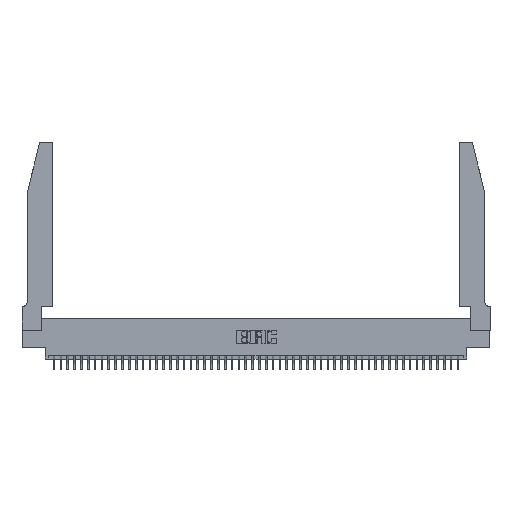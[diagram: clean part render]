
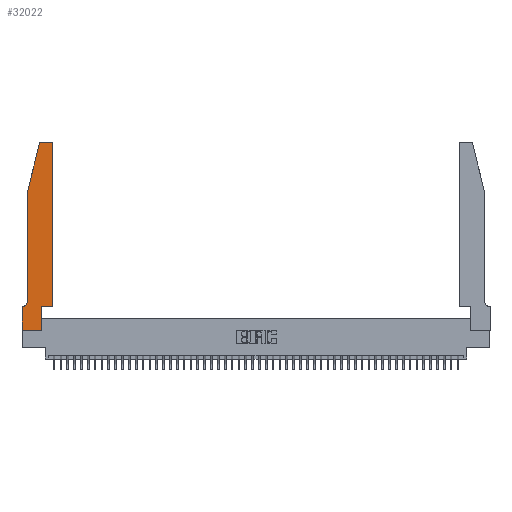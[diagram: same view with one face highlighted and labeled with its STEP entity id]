
A CAD part, top view. The second image highlights one B-rep face of the part: STEP entity #32022.
In plain terms, the highlighted planar face has unit normal (0, 0, 1).
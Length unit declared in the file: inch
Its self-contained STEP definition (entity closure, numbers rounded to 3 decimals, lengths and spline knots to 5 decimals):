
#297 = EDGE_CURVE ( 'NONE', #2750, #31447, #21843, .T. ) ;
#503 = CARTESIAN_POINT ( 'NONE',  ( 0., 0.35, 0.37 ) ) ;
#655 = ORIENTED_EDGE ( 'NONE', *, *, #27646, .T. ) ;
#872 = ORIENTED_EDGE ( 'NONE', *, *, #48148, .T. ) ;
#1070 = LINE ( 'NONE', #21088, #36600 ) ;
#2469 = EDGE_CURVE ( 'NONE', #24088, #16943, #8424, .T. ) ;
#2515 = CARTESIAN_POINT ( 'NONE',  ( 0.4505, 0.35, 0.37 ) ) ;
#2579 = AXIS2_PLACEMENT_3D ( 'NONE', #14143, #41237, #7570 ) ;
#2750 = VERTEX_POINT ( 'NONE', #43755 ) ;
#4694 = DIRECTION ( 'NONE',  ( 0., 0., 1. ) ) ;
#5607 = DIRECTION ( 'NONE',  ( 1., 0., 0. ) ) ;
#6545 = ORIENTED_EDGE ( 'NONE', *, *, #22013, .T. ) ;
#7570 = DIRECTION ( 'NONE',  ( -1., 0., 0. ) ) ;
#8029 = FACE_OUTER_BOUND ( 'NONE', #12773, .T. ) ;
#8160 = CARTESIAN_POINT ( 'NONE',  ( 0.0755, 2., 0.37 ) ) ;
#8228 = VERTEX_POINT ( 'NONE', #22815 ) ;
#8424 = CIRCLE ( 'NONE', #2579, 0.07 ) ;
#8636 = EDGE_CURVE ( 'NONE', #41171, #2750, #34935, .T. ) ;
#8825 = CARTESIAN_POINT ( 'NONE',  ( 0.4205, 2.72, 0.37 ) ) ;
#8946 = CARTESIAN_POINT ( 'NONE',  ( 0.2865, 0., 0.37 ) ) ;
#9603 = ORIENTED_EDGE ( 'NONE', *, *, #32944, .T. ) ;
#10611 = VECTOR ( 'NONE', #5607, 39.37008 ) ;
#10715 = CIRCLE ( 'NONE', #13180, 0.03 ) ;
#12484 = DIRECTION ( 'NONE',  ( 1., 0., 0. ) ) ;
#12741 = DIRECTION ( 'NONE',  ( 1., 0., 0. ) ) ;
#12773 = EDGE_LOOP ( 'NONE', ( #9603, #6545, #872, #45639, #31540, #655, #18144, #30575, #36050, #16463, #37172, #16275 ) ) ;
#13180 = AXIS2_PLACEMENT_3D ( 'NONE', #35712, #24237, #12484 ) ;
#13744 = VECTOR ( 'NONE', #36304, 39.37008 ) ;
#14143 = CARTESIAN_POINT ( 'NONE',  ( 0.0055, 0.42, 0.37 ) ) ;
#15810 = VECTOR ( 'NONE', #43331, 39.37008 ) ;
#15975 = DIRECTION ( 'NONE',  ( -1., 0., 0. ) ) ;
#16275 = ORIENTED_EDGE ( 'NONE', *, *, #45144, .T. ) ;
#16383 = CARTESIAN_POINT ( 'NONE',  ( 0., 0., 0.37 ) ) ;
#16463 = ORIENTED_EDGE ( 'NONE', *, *, #47046, .T. ) ;
#16923 = CARTESIAN_POINT ( 'NONE',  ( 0.4505, 0.35, 0.37 ) ) ;
#16943 = VERTEX_POINT ( 'NONE', #23658 ) ;
#17864 = LINE ( 'NONE', #47510, #33554 ) ;
#18144 = ORIENTED_EDGE ( 'NONE', *, *, #8636, .T. ) ;
#18869 = CARTESIAN_POINT ( 'NONE',  ( 0., 0.35, 0.37 ) ) ;
#20731 = CARTESIAN_POINT ( 'NONE',  ( 0.4505, 0.35, 0.37 ) ) ;
#21088 = CARTESIAN_POINT ( 'NONE',  ( 0.2605, 2.75, 0.37 ) ) ;
#21843 = LINE ( 'NONE', #16383, #15810 ) ;
#22013 = EDGE_CURVE ( 'NONE', #8228, #26638, #10715, .T. ) ;
#22389 = VERTEX_POINT ( 'NONE', #30265 ) ;
#22815 = CARTESIAN_POINT ( 'NONE',  ( 0.284, 2.75, 0.37 ) ) ;
#23383 = VECTOR ( 'NONE', #34622, 39.37008 ) ;
#23658 = CARTESIAN_POINT ( 'NONE',  ( 0.0055, 0.35, 0.37 ) ) ;
#24088 = VERTEX_POINT ( 'NONE', #38951 ) ;
#24237 = DIRECTION ( 'NONE',  ( 0., 0., 1. ) ) ;
#25683 = LINE ( 'NONE', #20731, #10611 ) ;
#26638 = VERTEX_POINT ( 'NONE', #29973 ) ;
#27556 = PLANE ( 'NONE',  #34699 ) ;
#27646 = EDGE_CURVE ( 'NONE', #16943, #41171, #32521, .T. ) ;
#28103 = VERTEX_POINT ( 'NONE', #2515 ) ;
#28664 = DIRECTION ( 'NONE',  ( 0., 1., 0. ) ) ;
#28729 = CARTESIAN_POINT ( 'NONE',  ( 0., 0., 0.37 ) ) ;
#29206 = DIRECTION ( 'NONE',  ( 0., -1., 0. ) ) ;
#29973 = CARTESIAN_POINT ( 'NONE',  ( 0.25487, 2.72718, 0.37 ) ) ;
#30004 = CARTESIAN_POINT ( 'NONE',  ( 0.0755, 2., 0.37 ) ) ;
#30265 = CARTESIAN_POINT ( 'NONE',  ( 0.4505, 2.72, 0.37 ) ) ;
#30575 = ORIENTED_EDGE ( 'NONE', *, *, #297, .T. ) ;
#31313 = VECTOR ( 'NONE', #15975, 39.37008 ) ;
#31447 = VERTEX_POINT ( 'NONE', #8946 ) ;
#31540 = ORIENTED_EDGE ( 'NONE', *, *, #2469, .T. ) ;
#31611 = CARTESIAN_POINT ( 'NONE',  ( 0.0755, 2., 0.37 ) ) ;
#32022 = ADVANCED_FACE ( 'NONE', ( #8029 ), #27556, .T. ) ;
#32082 = DIRECTION ( 'NONE',  ( -1., 0., 0. ) ) ;
#32521 = LINE ( 'NONE', #43116, #31313 ) ;
#32944 = EDGE_CURVE ( 'NONE', #43717, #8228, #1070, .T. ) ;
#33554 = VECTOR ( 'NONE', #28664, 39.37008 ) ;
#33805 = CIRCLE ( 'NONE', #40622, 0.03 ) ;
#34037 = VECTOR ( 'NONE', #36142, 39.37008 ) ;
#34622 = DIRECTION ( 'NONE',  ( 0., -1., 0. ) ) ;
#34699 = AXIS2_PLACEMENT_3D ( 'NONE', #503, #4694, #46423 ) ;
#34935 = LINE ( 'NONE', #28729, #48744 ) ;
#35712 = CARTESIAN_POINT ( 'NONE',  ( 0.284, 2.72, 0.37 ) ) ;
#35794 = DIRECTION ( 'NONE',  ( 0., 0., 1. ) ) ;
#36050 = ORIENTED_EDGE ( 'NONE', *, *, #46980, .T. ) ;
#36084 = LINE ( 'NONE', #8160, #23383 ) ;
#36142 = DIRECTION ( 'NONE',  ( -0.239, -0.971, 0. ) ) ;
#36304 = DIRECTION ( 'NONE',  ( 0., 1., 0. ) ) ;
#36600 = VECTOR ( 'NONE', #32082, 39.37008 ) ;
#37172 = ORIENTED_EDGE ( 'NONE', *, *, #46386, .T. ) ;
#38293 = EDGE_CURVE ( 'NONE', #49750, #24088, #36084, .T. ) ;
#38951 = CARTESIAN_POINT ( 'NONE',  ( 0.0755, 0.42, 0.37 ) ) ;
#40622 = AXIS2_PLACEMENT_3D ( 'NONE', #8825, #35794, #12741 ) ;
#41171 = VERTEX_POINT ( 'NONE', #18869 ) ;
#41237 = DIRECTION ( 'NONE',  ( 0., 0., -1. ) ) ;
#42665 = LINE ( 'NONE', #16923, #13744 ) ;
#43116 = CARTESIAN_POINT ( 'NONE',  ( 0.0755, 0.35, 0.37 ) ) ;
#43331 = DIRECTION ( 'NONE',  ( 1., 0., 0. ) ) ;
#43717 = VERTEX_POINT ( 'NONE', #45992 ) ;
#43755 = CARTESIAN_POINT ( 'NONE',  ( 0., 0., 0.37 ) ) ;
#44283 = LINE ( 'NONE', #31611, #34037 ) ;
#44827 = CARTESIAN_POINT ( 'NONE',  ( 0.2865, 0.35, 0.37 ) ) ;
#45144 = EDGE_CURVE ( 'NONE', #22389, #43717, #33805, .T. ) ;
#45639 = ORIENTED_EDGE ( 'NONE', *, *, #38293, .T. ) ;
#45992 = CARTESIAN_POINT ( 'NONE',  ( 0.4205, 2.75, 0.37 ) ) ;
#46386 = EDGE_CURVE ( 'NONE', #28103, #22389, #42665, .T. ) ;
#46423 = DIRECTION ( 'NONE',  ( 1., 0., 0. ) ) ;
#46980 = EDGE_CURVE ( 'NONE', #31447, #48505, #17864, .T. ) ;
#47046 = EDGE_CURVE ( 'NONE', #48505, #28103, #25683, .T. ) ;
#47510 = CARTESIAN_POINT ( 'NONE',  ( 0.2865, 0.35, 0.37 ) ) ;
#48148 = EDGE_CURVE ( 'NONE', #26638, #49750, #44283, .T. ) ;
#48505 = VERTEX_POINT ( 'NONE', #44827 ) ;
#48744 = VECTOR ( 'NONE', #29206, 39.37008 ) ;
#49750 = VERTEX_POINT ( 'NONE', #30004 ) ;
